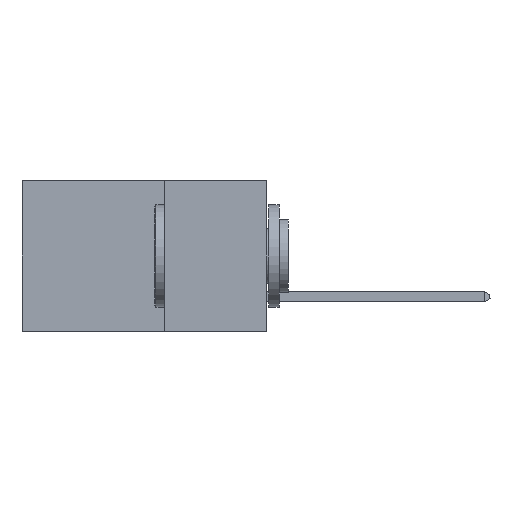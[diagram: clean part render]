
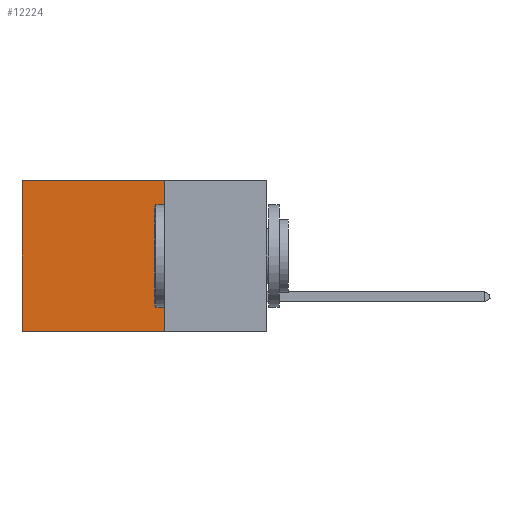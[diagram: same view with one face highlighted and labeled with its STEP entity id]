
A CAD part, left-side view. The second image highlights one B-rep face of the part: STEP entity #12224.
In plain terms, the highlighted planar face has unit normal (-1, 0, 0).
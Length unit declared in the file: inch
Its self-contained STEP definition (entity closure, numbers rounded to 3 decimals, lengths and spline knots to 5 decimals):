
#8 = VERTEX_POINT ( 'NONE', #13077 ) ;
#483 = VERTEX_POINT ( 'NONE', #45007 ) ;
#1148 = CARTESIAN_POINT ( 'NONE',  ( 0.2875, 0.25, -0.37 ) ) ;
#2010 = CARTESIAN_POINT ( 'NONE',  ( 0.2875, 0.25, 0. ) ) ;
#4011 = LINE ( 'NONE', #1148, #33177 ) ;
#4188 = EDGE_CURVE ( 'NONE', #8, #35084, #33091, .T. ) ;
#4380 = AXIS2_PLACEMENT_3D ( 'NONE', #30509, #23731, #30818 ) ;
#4561 = DIRECTION ( 'NONE',  ( 0., 0., -1. ) ) ;
#4614 = ORIENTED_EDGE ( 'NONE', *, *, #4188, .T. ) ;
#8056 = DIRECTION ( 'NONE',  ( 0., 1., 0. ) ) ;
#8884 = VECTOR ( 'NONE', #4561, 39.37008 ) ;
#12224 = ADVANCED_FACE ( 'NONE', ( #46423 ), #27330, .F. ) ;
#12279 = CARTESIAN_POINT ( 'NONE',  ( 0.2875, 0.6, 0. ) ) ;
#12694 = DIRECTION ( 'NONE',  ( 0., 0., -1. ) ) ;
#13077 = CARTESIAN_POINT ( 'NONE',  ( 0.2875, 0.25, 0. ) ) ;
#13101 = EDGE_CURVE ( 'NONE', #8, #483, #45789, .T. ) ;
#15414 = VERTEX_POINT ( 'NONE', #40983 ) ;
#18388 = LINE ( 'NONE', #43961, #8884 ) ;
#19994 = CARTESIAN_POINT ( 'NONE',  ( 0.2875, 0.25, 0. ) ) ;
#21072 = ORIENTED_EDGE ( 'NONE', *, *, #13101, .F. ) ;
#21235 = ORIENTED_EDGE ( 'NONE', *, *, #45188, .F. ) ;
#23731 = DIRECTION ( 'NONE',  ( 1., 0., 0. ) ) ;
#26625 = EDGE_CURVE ( 'NONE', #35084, #15414, #18388, .T. ) ;
#27330 = PLANE ( 'NONE',  #4380 ) ;
#27999 = EDGE_LOOP ( 'NONE', ( #46023, #21235, #21072, #4614 ) ) ;
#30266 = VECTOR ( 'NONE', #34298, 39.37008 ) ;
#30509 = CARTESIAN_POINT ( 'NONE',  ( 0.2875, 0.25, 0. ) ) ;
#30818 = DIRECTION ( 'NONE',  ( 0., 0., -1. ) ) ;
#33091 = LINE ( 'NONE', #2010, #30266 ) ;
#33177 = VECTOR ( 'NONE', #8056, 39.37008 ) ;
#34298 = DIRECTION ( 'NONE',  ( 0., 1., 0. ) ) ;
#35084 = VERTEX_POINT ( 'NONE', #12279 ) ;
#40983 = CARTESIAN_POINT ( 'NONE',  ( 0.2875, 0.6, -0.37 ) ) ;
#43961 = CARTESIAN_POINT ( 'NONE',  ( 0.2875, 0.6, 0. ) ) ;
#45007 = CARTESIAN_POINT ( 'NONE',  ( 0.2875, 0.25, -0.37 ) ) ;
#45188 = EDGE_CURVE ( 'NONE', #483, #15414, #4011, .T. ) ;
#45789 = LINE ( 'NONE', #19994, #46336 ) ;
#46023 = ORIENTED_EDGE ( 'NONE', *, *, #26625, .T. ) ;
#46336 = VECTOR ( 'NONE', #12694, 39.37008 ) ;
#46423 = FACE_OUTER_BOUND ( 'NONE', #27999, .T. ) ;
